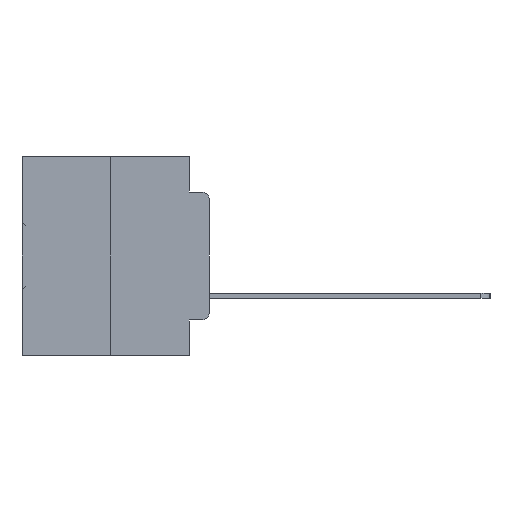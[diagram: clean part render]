
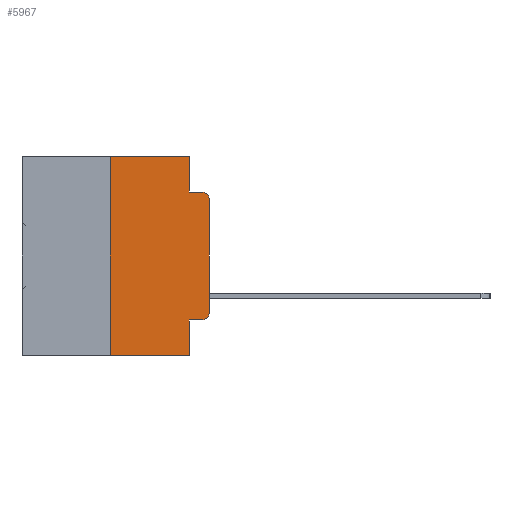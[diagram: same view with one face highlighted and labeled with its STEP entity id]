
A CAD part, left-side view. The second image highlights one B-rep face of the part: STEP entity #5967.
In plain terms, the highlighted planar face has unit normal (-1, 0, 0).
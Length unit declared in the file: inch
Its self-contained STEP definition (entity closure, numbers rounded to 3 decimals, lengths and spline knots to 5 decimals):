
#27 = ORIENTED_EDGE ( 'NONE', *, *, #28914, .F. ) ;
#52 = ORIENTED_EDGE ( 'NONE', *, *, #16282, .T. ) ;
#113 = VECTOR ( 'NONE', #17505, 39.37008 ) ;
#231 = AXIS2_PLACEMENT_3D ( 'NONE', #5657, #13938, #32789 ) ;
#449 = ORIENTED_EDGE ( 'NONE', *, *, #34946, .T. ) ;
#1512 = CARTESIAN_POINT ( 'NONE',  ( 0., 0.051, -0.0885 ) ) ;
#1620 = CARTESIAN_POINT ( 'NONE',  ( 0., 0.051, 0. ) ) ;
#1784 = DIRECTION ( 'NONE',  ( -1., 0., 0. ) ) ;
#4195 = DIRECTION ( 'NONE',  ( -1., 0., 0. ) ) ;
#4543 = DIRECTION ( 'NONE',  ( 0., 0., 1. ) ) ;
#4583 = CARTESIAN_POINT ( 'NONE',  ( 0., 0.051, 0. ) ) ;
#4887 = VECTOR ( 'NONE', #20960, 39.37008 ) ;
#5657 = CARTESIAN_POINT ( 'NONE',  ( 0., 0.473, 0. ) ) ;
#5782 = DIRECTION ( 'NONE',  ( 0., -1., 0. ) ) ;
#5807 = LINE ( 'NONE', #33637, #113 ) ;
#5967 = ADVANCED_FACE ( 'NONE', ( #17001 ), #30069, .F. ) ;
#6332 = VECTOR ( 'NONE', #15468, 39.37008 ) ;
#6641 = VERTEX_POINT ( 'NONE', #14123 ) ;
#6731 = VECTOR ( 'NONE', #22791, 39.37008 ) ;
#7813 = EDGE_CURVE ( 'NONE', #9803, #13709, #29490, .T. ) ;
#7907 = VECTOR ( 'NONE', #5782, 39.37008 ) ;
#8441 = CARTESIAN_POINT ( 'NONE',  ( 0., 0., -0.1085 ) ) ;
#9803 = VERTEX_POINT ( 'NONE', #30484 ) ;
#10087 = EDGE_CURVE ( 'NONE', #13709, #26936, #34579, .T. ) ;
#10175 = VERTEX_POINT ( 'NONE', #26628 ) ;
#11482 = ORIENTED_EDGE ( 'NONE', *, *, #10087, .F. ) ;
#12395 = ORIENTED_EDGE ( 'NONE', *, *, #15591, .F. ) ;
#12813 = CARTESIAN_POINT ( 'NONE',  ( 0., 0., 0. ) ) ;
#13709 = VERTEX_POINT ( 'NONE', #15871 ) ;
#13938 = DIRECTION ( 'NONE',  ( 1., 0., 0. ) ) ;
#13945 = CARTESIAN_POINT ( 'NONE',  ( 0., 0.473, 0. ) ) ;
#14123 = CARTESIAN_POINT ( 'NONE',  ( 0., 0.25, -0.5 ) ) ;
#14785 = ORIENTED_EDGE ( 'NONE', *, *, #30685, .F. ) ;
#15167 = VECTOR ( 'NONE', #23546, 39.37008 ) ;
#15249 = ORIENTED_EDGE ( 'NONE', *, *, #7813, .F. ) ;
#15468 = DIRECTION ( 'NONE',  ( 0., -1., 0. ) ) ;
#15591 = EDGE_CURVE ( 'NONE', #26936, #19117, #5807, .T. ) ;
#15871 = CARTESIAN_POINT ( 'NONE',  ( 0., 0.051, 0. ) ) ;
#16018 = LINE ( 'NONE', #12813, #22368 ) ;
#16282 = EDGE_CURVE ( 'NONE', #25132, #31157, #29198, .T. ) ;
#16515 = ORIENTED_EDGE ( 'NONE', *, *, #22850, .T. ) ;
#17001 = FACE_OUTER_BOUND ( 'NONE', #25704, .T. ) ;
#17505 = DIRECTION ( 'NONE',  ( 0., -1., 0. ) ) ;
#18246 = CARTESIAN_POINT ( 'NONE',  ( 0., 0.02, -0.1085 ) ) ;
#18251 = DIRECTION ( 'NONE',  ( 0., 0., 1. ) ) ;
#18678 = ORIENTED_EDGE ( 'NONE', *, *, #33799, .T. ) ;
#19091 = CIRCLE ( 'NONE', #28376, 0.02 ) ;
#19117 = VERTEX_POINT ( 'NONE', #33017 ) ;
#20524 = LINE ( 'NONE', #31611, #26862 ) ;
#20583 = CARTESIAN_POINT ( 'NONE',  ( 0., 0.02, -0.3915 ) ) ;
#20960 = DIRECTION ( 'NONE',  ( 0., 0., -1. ) ) ;
#20966 = DIRECTION ( 'NONE',  ( 0., 0., -1. ) ) ;
#22368 = VECTOR ( 'NONE', #18251, 39.37008 ) ;
#22791 = DIRECTION ( 'NONE',  ( 0., -1., 0. ) ) ;
#22850 = EDGE_CURVE ( 'NONE', #31057, #19117, #24180, .T. ) ;
#23328 = DIRECTION ( 'NONE',  ( 0., 0., -1. ) ) ;
#23546 = DIRECTION ( 'NONE',  ( 0., 0., -1. ) ) ;
#24180 = CIRCLE ( 'NONE', #26340, 0.02 ) ;
#24641 = EDGE_CURVE ( 'NONE', #10175, #31057, #16018, .T. ) ;
#25132 = VERTEX_POINT ( 'NONE', #31143 ) ;
#25257 = CARTESIAN_POINT ( 'NONE',  ( 0., 0.02, -0.4115 ) ) ;
#25498 = CARTESIAN_POINT ( 'NONE',  ( 0., 0.051, -0.4115 ) ) ;
#25704 = EDGE_LOOP ( 'NONE', ( #25910, #16515, #12395, #11482, #15249, #14785, #18678, #27, #52, #449 ) ) ;
#25910 = ORIENTED_EDGE ( 'NONE', *, *, #24641, .T. ) ;
#26336 = CARTESIAN_POINT ( 'NONE',  ( 0., 0.473, -0.5 ) ) ;
#26340 = AXIS2_PLACEMENT_3D ( 'NONE', #18246, #1784, #20966 ) ;
#26628 = CARTESIAN_POINT ( 'NONE',  ( 0., 0., -0.3915 ) ) ;
#26862 = VECTOR ( 'NONE', #4543, 39.37008 ) ;
#26936 = VERTEX_POINT ( 'NONE', #1512 ) ;
#27990 = LINE ( 'NONE', #26336, #6332 ) ;
#28376 = AXIS2_PLACEMENT_3D ( 'NONE', #20583, #4195, #23328 ) ;
#28672 = LINE ( 'NONE', #1620, #15167 ) ;
#28914 = EDGE_CURVE ( 'NONE', #25132, #30442, #28672, .T. ) ;
#29198 = LINE ( 'NONE', #25498, #6731 ) ;
#29490 = LINE ( 'NONE', #13945, #7907 ) ;
#30069 = PLANE ( 'NONE',  #231 ) ;
#30442 = VERTEX_POINT ( 'NONE', #30443 ) ;
#30443 = CARTESIAN_POINT ( 'NONE',  ( 0., 0.051, -0.5 ) ) ;
#30484 = CARTESIAN_POINT ( 'NONE',  ( 0., 0.25, 0. ) ) ;
#30685 = EDGE_CURVE ( 'NONE', #6641, #9803, #20524, .T. ) ;
#31057 = VERTEX_POINT ( 'NONE', #8441 ) ;
#31143 = CARTESIAN_POINT ( 'NONE',  ( 0., 0.051, -0.4115 ) ) ;
#31157 = VERTEX_POINT ( 'NONE', #25257 ) ;
#31611 = CARTESIAN_POINT ( 'NONE',  ( 0., 0.25, 0. ) ) ;
#32789 = DIRECTION ( 'NONE',  ( 0., 0., -1. ) ) ;
#33017 = CARTESIAN_POINT ( 'NONE',  ( 0., 0.02, -0.0885 ) ) ;
#33637 = CARTESIAN_POINT ( 'NONE',  ( 0., 0.051, -0.0885 ) ) ;
#33799 = EDGE_CURVE ( 'NONE', #6641, #30442, #27990, .T. ) ;
#34579 = LINE ( 'NONE', #4583, #4887 ) ;
#34946 = EDGE_CURVE ( 'NONE', #31157, #10175, #19091, .T. ) ;
